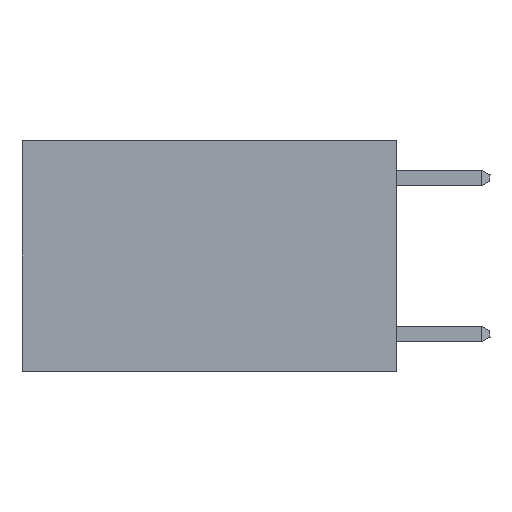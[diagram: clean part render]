
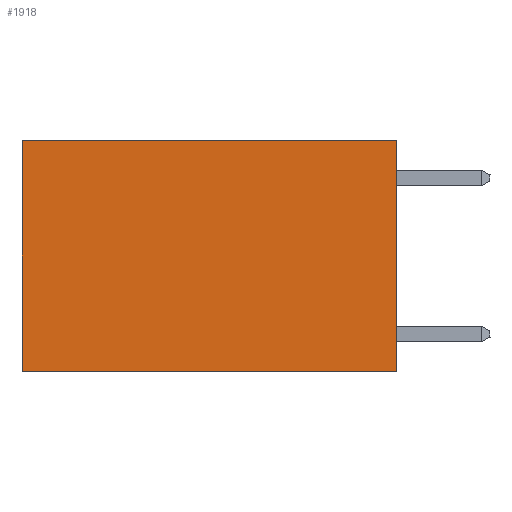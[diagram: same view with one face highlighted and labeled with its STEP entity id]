
A CAD part, left-side view. The second image highlights one B-rep face of the part: STEP entity #1918.
In plain terms, the highlighted planar face has unit normal (-1, 0, 0).
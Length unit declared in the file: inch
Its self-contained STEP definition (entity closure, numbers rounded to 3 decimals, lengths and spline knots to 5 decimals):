
#369 = VERTEX_POINT ( 'NONE', #4689 ) ;
#846 = LINE ( 'NONE', #6126, #3772 ) ;
#895 = ORIENTED_EDGE ( 'NONE', *, *, #8248, .T. ) ;
#1027 = LINE ( 'NONE', #6440, #4962 ) ;
#1518 = DIRECTION ( 'NONE',  ( 0., 0., -1. ) ) ;
#1763 = DIRECTION ( 'NONE',  ( 0., 1., 0. ) ) ;
#1918 = ADVANCED_FACE ( 'NONE', ( #13421 ), #9035, .F. ) ;
#2054 = VERTEX_POINT ( 'NONE', #12141 ) ;
#2300 = VECTOR ( 'NONE', #9278, 39.37008 ) ;
#2595 = AXIS2_PLACEMENT_3D ( 'NONE', #4504, #11186, #3228 ) ;
#2870 = LINE ( 'NONE', #4898, #2300 ) ;
#2952 = ORIENTED_EDGE ( 'NONE', *, *, #3929, .F. ) ;
#3228 = DIRECTION ( 'NONE',  ( 0., 0., -1. ) ) ;
#3772 = VECTOR ( 'NONE', #1518, 39.37008 ) ;
#3929 = EDGE_CURVE ( 'NONE', #2054, #5577, #846, .T. ) ;
#4368 = EDGE_CURVE ( 'NONE', #5577, #11643, #6320, .T. ) ;
#4504 = CARTESIAN_POINT ( 'NONE',  ( 0.2625, 0., 0. ) ) ;
#4689 = CARTESIAN_POINT ( 'NONE',  ( 0.2625, 0.6, 0. ) ) ;
#4898 = CARTESIAN_POINT ( 'NONE',  ( 0.2625, 0.6, 0. ) ) ;
#4962 = VECTOR ( 'NONE', #11951, 39.37008 ) ;
#5577 = VERTEX_POINT ( 'NONE', #7031 ) ;
#6126 = CARTESIAN_POINT ( 'NONE',  ( 0.2625, 0., 0. ) ) ;
#6320 = LINE ( 'NONE', #12863, #11339 ) ;
#6440 = CARTESIAN_POINT ( 'NONE',  ( 0.2625, 0., 0. ) ) ;
#7031 = CARTESIAN_POINT ( 'NONE',  ( 0.2625, 0., -0.37 ) ) ;
#8248 = EDGE_CURVE ( 'NONE', #2054, #369, #1027, .T. ) ;
#8946 = ORIENTED_EDGE ( 'NONE', *, *, #13476, .T. ) ;
#9035 = PLANE ( 'NONE',  #2595 ) ;
#9269 = CARTESIAN_POINT ( 'NONE',  ( 0.2625, 0.6, -0.37 ) ) ;
#9278 = DIRECTION ( 'NONE',  ( 0., 0., -1. ) ) ;
#11186 = DIRECTION ( 'NONE',  ( 1., 0., 0. ) ) ;
#11339 = VECTOR ( 'NONE', #1763, 39.37008 ) ;
#11643 = VERTEX_POINT ( 'NONE', #9269 ) ;
#11951 = DIRECTION ( 'NONE',  ( 0., 1., 0. ) ) ;
#12049 = ORIENTED_EDGE ( 'NONE', *, *, #4368, .F. ) ;
#12141 = CARTESIAN_POINT ( 'NONE',  ( 0.2625, 0., 0. ) ) ;
#12171 = EDGE_LOOP ( 'NONE', ( #8946, #12049, #2952, #895 ) ) ;
#12863 = CARTESIAN_POINT ( 'NONE',  ( 0.2625, 0., -0.37 ) ) ;
#13421 = FACE_OUTER_BOUND ( 'NONE', #12171, .T. ) ;
#13476 = EDGE_CURVE ( 'NONE', #369, #11643, #2870, .T. ) ;
